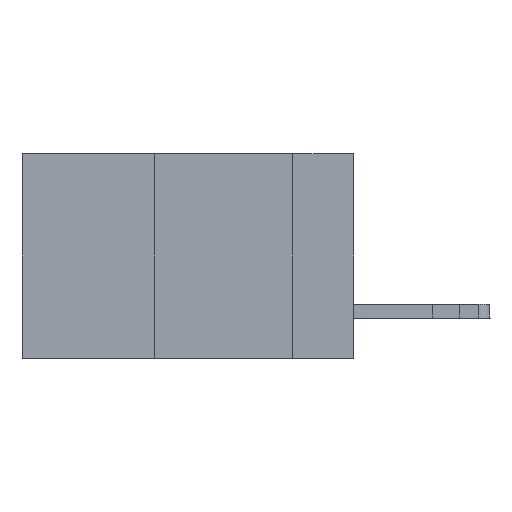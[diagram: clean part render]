
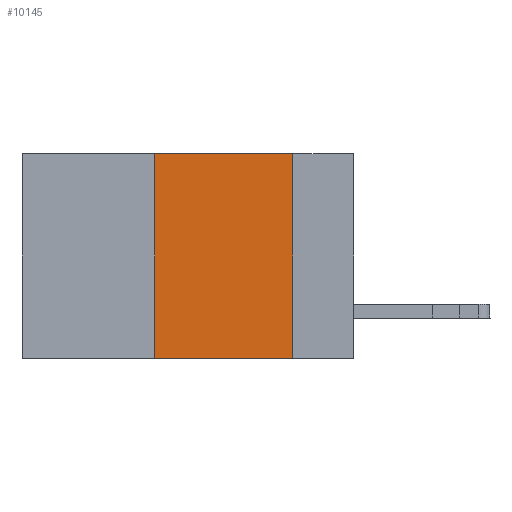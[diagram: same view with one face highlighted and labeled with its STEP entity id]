
A CAD part, left-side view. The second image highlights one B-rep face of the part: STEP entity #10145.
In plain terms, the highlighted planar face has unit normal (-1, 0, 0).
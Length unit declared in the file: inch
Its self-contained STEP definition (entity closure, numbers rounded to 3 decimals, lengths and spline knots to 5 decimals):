
#1932 = VECTOR ( 'NONE', #6785, 39.37008 ) ;
#3291 = PLANE ( 'NONE',  #6998 ) ;
#3715 = CARTESIAN_POINT ( 'NONE',  ( 0., 0.36, 0. ) ) ;
#4124 = EDGE_CURVE ( 'NONE', #13008, #18266, #19256, .T. ) ;
#4217 = EDGE_LOOP ( 'NONE', ( #5537, #19606, #9465, #20769 ) ) ;
#4272 = CARTESIAN_POINT ( 'NONE',  ( 0., 0.36, -0.37 ) ) ;
#4289 = EDGE_CURVE ( 'NONE', #19130, #20892, #20483, .T. ) ;
#4332 = DIRECTION ( 'NONE',  ( 0., -1., 0. ) ) ;
#4712 = CARTESIAN_POINT ( 'NONE',  ( 0., 0.6, -0.37 ) ) ;
#5537 = ORIENTED_EDGE ( 'NONE', *, *, #13391, .F. ) ;
#6482 = VECTOR ( 'NONE', #13583, 39.37008 ) ;
#6739 = DIRECTION ( 'NONE',  ( 0., 0., -1. ) ) ;
#6785 = DIRECTION ( 'NONE',  ( 0., -1., 0. ) ) ;
#6809 = CARTESIAN_POINT ( 'NONE',  ( 0., 0.6, 0. ) ) ;
#6998 = AXIS2_PLACEMENT_3D ( 'NONE', #8398, #16743, #6739 ) ;
#8159 = CARTESIAN_POINT ( 'NONE',  ( 0., 0.11, 0. ) ) ;
#8398 = CARTESIAN_POINT ( 'NONE',  ( 0., 0.6, 0. ) ) ;
#8812 = CARTESIAN_POINT ( 'NONE',  ( 0., 0.11, 0. ) ) ;
#8893 = EDGE_CURVE ( 'NONE', #19130, #13008, #11013, .T. ) ;
#9465 = ORIENTED_EDGE ( 'NONE', *, *, #8893, .F. ) ;
#10145 = ADVANCED_FACE ( 'NONE', ( #19684 ), #3291, .F. ) ;
#11013 = LINE ( 'NONE', #21643, #6482 ) ;
#12202 = CARTESIAN_POINT ( 'NONE',  ( 0., 0.11, -0.37 ) ) ;
#13008 = VERTEX_POINT ( 'NONE', #3715 ) ;
#13223 = DIRECTION ( 'NONE',  ( 0., 0., -1. ) ) ;
#13391 = EDGE_CURVE ( 'NONE', #18266, #20892, #15447, .T. ) ;
#13583 = DIRECTION ( 'NONE',  ( 0., 0., 1. ) ) ;
#15447 = LINE ( 'NONE', #8159, #19283 ) ;
#16200 = VECTOR ( 'NONE', #4332, 39.37008 ) ;
#16743 = DIRECTION ( 'NONE',  ( 1., 0., 0. ) ) ;
#18266 = VERTEX_POINT ( 'NONE', #8812 ) ;
#19130 = VERTEX_POINT ( 'NONE', #4272 ) ;
#19256 = LINE ( 'NONE', #6809, #1932 ) ;
#19283 = VECTOR ( 'NONE', #13223, 39.37008 ) ;
#19606 = ORIENTED_EDGE ( 'NONE', *, *, #4124, .F. ) ;
#19684 = FACE_OUTER_BOUND ( 'NONE', #4217, .T. ) ;
#20483 = LINE ( 'NONE', #4712, #16200 ) ;
#20769 = ORIENTED_EDGE ( 'NONE', *, *, #4289, .T. ) ;
#20892 = VERTEX_POINT ( 'NONE', #12202 ) ;
#21643 = CARTESIAN_POINT ( 'NONE',  ( 0., 0.36, 0. ) ) ;
